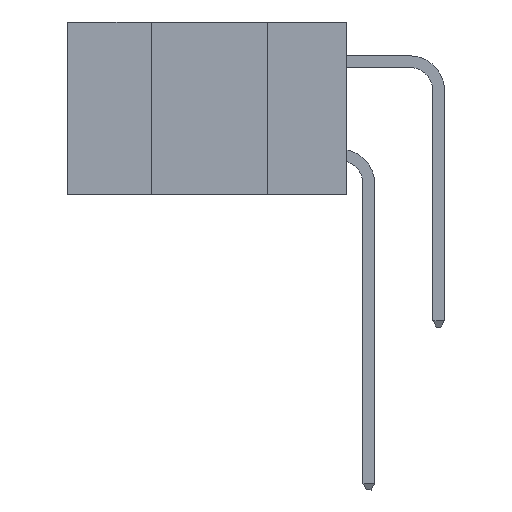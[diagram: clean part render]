
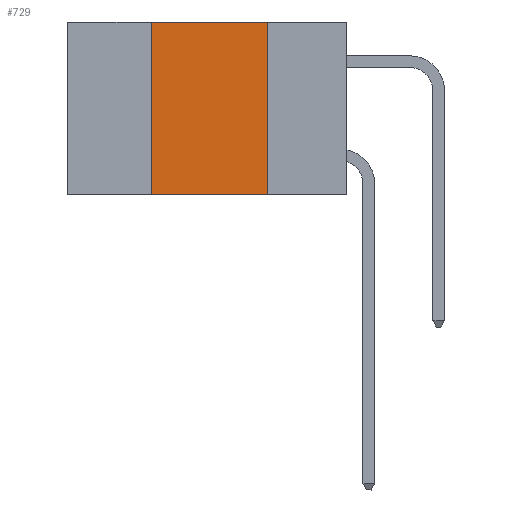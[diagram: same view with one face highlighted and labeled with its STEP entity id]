
A CAD part, left-side view. The second image highlights one B-rep face of the part: STEP entity #729.
In plain terms, the highlighted planar face has unit normal (-1, 0, 0).
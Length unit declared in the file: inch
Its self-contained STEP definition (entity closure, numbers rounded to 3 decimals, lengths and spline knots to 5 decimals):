
#178 = ORIENTED_EDGE ( 'NONE', *, *, #17107, .F. ) ;
#729 = ADVANCED_FACE ( 'NONE', ( #18252 ), #5104, .F. ) ;
#856 = LINE ( 'NONE', #3001, #23935 ) ;
#2348 = ORIENTED_EDGE ( 'NONE', *, *, #15289, .F. ) ;
#2427 = VERTEX_POINT ( 'NONE', #16885 ) ;
#3001 = CARTESIAN_POINT ( 'NONE',  ( 0., 0.17, 0. ) ) ;
#3287 = LINE ( 'NONE', #11572, #18208 ) ;
#5104 = PLANE ( 'NONE',  #11248 ) ;
#5206 = CARTESIAN_POINT ( 'NONE',  ( 0., 0.42, 0. ) ) ;
#5453 = CARTESIAN_POINT ( 'NONE',  ( 0., 0.17, 0. ) ) ;
#5584 = VERTEX_POINT ( 'NONE', #20700 ) ;
#5627 = VECTOR ( 'NONE', #21578, 39.37008 ) ;
#5704 = DIRECTION ( 'NONE',  ( 0., -1., 0. ) ) ;
#7496 = DIRECTION ( 'NONE',  ( 0., -1., 0. ) ) ;
#10277 = DIRECTION ( 'NONE',  ( 1., 0., 0. ) ) ;
#10404 = DIRECTION ( 'NONE',  ( 0., 0., -1. ) ) ;
#11248 = AXIS2_PLACEMENT_3D ( 'NONE', #14338, #10277, #10404 ) ;
#11572 = CARTESIAN_POINT ( 'NONE',  ( 0., 0.6, -0.37 ) ) ;
#12006 = ORIENTED_EDGE ( 'NONE', *, *, #13201, .F. ) ;
#13201 = EDGE_CURVE ( 'NONE', #2427, #5584, #23474, .T. ) ;
#14338 = CARTESIAN_POINT ( 'NONE',  ( 0., 0.6, 0. ) ) ;
#15244 = VECTOR ( 'NONE', #5704, 39.37008 ) ;
#15289 = EDGE_CURVE ( 'NONE', #5584, #20215, #18153, .T. ) ;
#16885 = CARTESIAN_POINT ( 'NONE',  ( 0., 0.42, -0.37 ) ) ;
#17107 = EDGE_CURVE ( 'NONE', #20215, #17705, #856, .T. ) ;
#17705 = VERTEX_POINT ( 'NONE', #18371 ) ;
#17754 = DIRECTION ( 'NONE',  ( 0., 0., -1. ) ) ;
#18153 = LINE ( 'NONE', #22356, #15244 ) ;
#18208 = VECTOR ( 'NONE', #7496, 39.37008 ) ;
#18252 = FACE_OUTER_BOUND ( 'NONE', #23063, .T. ) ;
#18371 = CARTESIAN_POINT ( 'NONE',  ( 0., 0.17, -0.37 ) ) ;
#20215 = VERTEX_POINT ( 'NONE', #5453 ) ;
#20700 = CARTESIAN_POINT ( 'NONE',  ( 0., 0.42, 0. ) ) ;
#21569 = EDGE_CURVE ( 'NONE', #2427, #17705, #3287, .T. ) ;
#21578 = DIRECTION ( 'NONE',  ( 0., 0., 1. ) ) ;
#22356 = CARTESIAN_POINT ( 'NONE',  ( 0., 0.6, 0. ) ) ;
#23063 = EDGE_LOOP ( 'NONE', ( #178, #2348, #12006, #23557 ) ) ;
#23474 = LINE ( 'NONE', #5206, #5627 ) ;
#23557 = ORIENTED_EDGE ( 'NONE', *, *, #21569, .T. ) ;
#23935 = VECTOR ( 'NONE', #17754, 39.37008 ) ;
